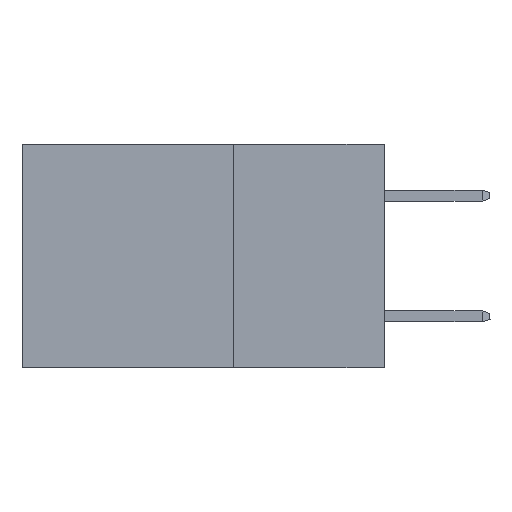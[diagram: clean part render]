
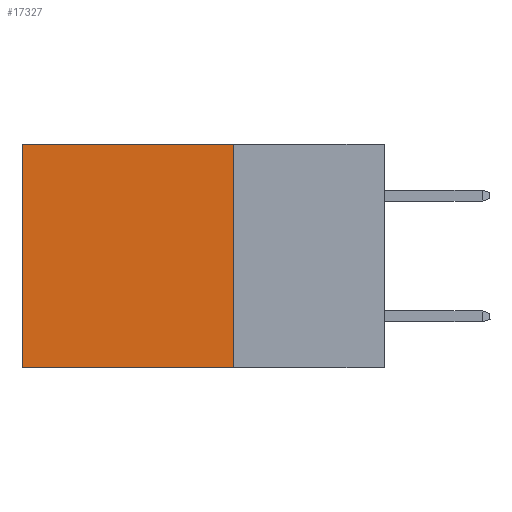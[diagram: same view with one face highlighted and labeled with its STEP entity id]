
A CAD part, left-side view. The second image highlights one B-rep face of the part: STEP entity #17327.
In plain terms, the highlighted planar face has unit normal (-1, 0, 0).
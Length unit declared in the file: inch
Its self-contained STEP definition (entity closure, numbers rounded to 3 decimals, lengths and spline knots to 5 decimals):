
#77 = AXIS2_PLACEMENT_3D ( 'NONE', #21028, #17389, #5917 ) ;
#150 = CARTESIAN_POINT ( 'NONE',  ( 0.2615, 0.25, -0.37 ) ) ;
#1194 = VERTEX_POINT ( 'NONE', #15912 ) ;
#3439 = CARTESIAN_POINT ( 'NONE',  ( 0.2615, 0.6, 0. ) ) ;
#5917 = DIRECTION ( 'NONE',  ( 0., 0., -1. ) ) ;
#6701 = EDGE_CURVE ( 'NONE', #14339, #1194, #14831, .T. ) ;
#7060 = VERTEX_POINT ( 'NONE', #150 ) ;
#7778 = DIRECTION ( 'NONE',  ( 0., 1., 0. ) ) ;
#8293 = ORIENTED_EDGE ( 'NONE', *, *, #6701, .T. ) ;
#8931 = CARTESIAN_POINT ( 'NONE',  ( 0.2615, 0.6, -0.37 ) ) ;
#9728 = EDGE_CURVE ( 'NONE', #7060, #1194, #18294, .T. ) ;
#9812 = VECTOR ( 'NONE', #16578, 39.37008 ) ;
#10406 = LINE ( 'NONE', #18478, #12645 ) ;
#10664 = VECTOR ( 'NONE', #21515, 39.37008 ) ;
#11255 = LINE ( 'NONE', #12168, #10664 ) ;
#11607 = CARTESIAN_POINT ( 'NONE',  ( 0.2615, 0.25, -0.37 ) ) ;
#12168 = CARTESIAN_POINT ( 'NONE',  ( 0.2615, 0.25, -0.37 ) ) ;
#12645 = VECTOR ( 'NONE', #20331, 39.37008 ) ;
#13280 = VECTOR ( 'NONE', #7778, 39.37008 ) ;
#14339 = VERTEX_POINT ( 'NONE', #3439 ) ;
#14831 = LINE ( 'NONE', #8931, #9812 ) ;
#15409 = EDGE_CURVE ( 'NONE', #21227, #7060, #11255, .T. ) ;
#15486 = PLANE ( 'NONE',  #77 ) ;
#15584 = ORIENTED_EDGE ( 'NONE', *, *, #9728, .F. ) ;
#15912 = CARTESIAN_POINT ( 'NONE',  ( 0.2615, 0.6, -0.37 ) ) ;
#16336 = EDGE_CURVE ( 'NONE', #21227, #14339, #10406, .T. ) ;
#16578 = DIRECTION ( 'NONE',  ( 0., 0., -1. ) ) ;
#17274 = EDGE_LOOP ( 'NONE', ( #8293, #15584, #21086, #18237 ) ) ;
#17327 = ADVANCED_FACE ( 'NONE', ( #22968 ), #15486, .F. ) ;
#17389 = DIRECTION ( 'NONE',  ( 1., 0., 0. ) ) ;
#18237 = ORIENTED_EDGE ( 'NONE', *, *, #16336, .T. ) ;
#18294 = LINE ( 'NONE', #11607, #13280 ) ;
#18478 = CARTESIAN_POINT ( 'NONE',  ( 0.2615, 0.25, 0. ) ) ;
#18673 = CARTESIAN_POINT ( 'NONE',  ( 0.2615, 0.25, 0. ) ) ;
#20331 = DIRECTION ( 'NONE',  ( 0., 1., 0. ) ) ;
#21028 = CARTESIAN_POINT ( 'NONE',  ( 0.2615, 0.25, -0.37 ) ) ;
#21086 = ORIENTED_EDGE ( 'NONE', *, *, #15409, .F. ) ;
#21227 = VERTEX_POINT ( 'NONE', #18673 ) ;
#21515 = DIRECTION ( 'NONE',  ( 0., 0., -1. ) ) ;
#22968 = FACE_OUTER_BOUND ( 'NONE', #17274, .T. ) ;
